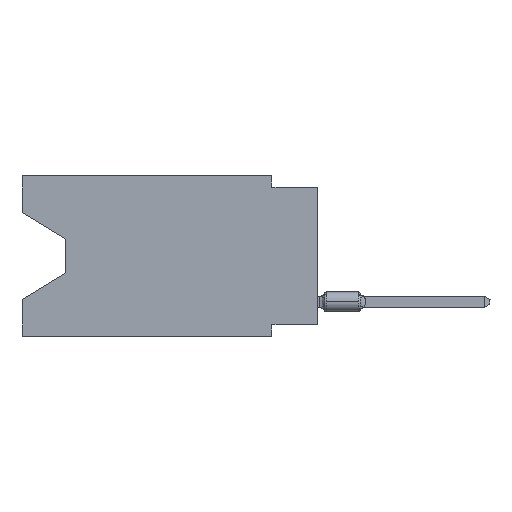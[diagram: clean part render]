
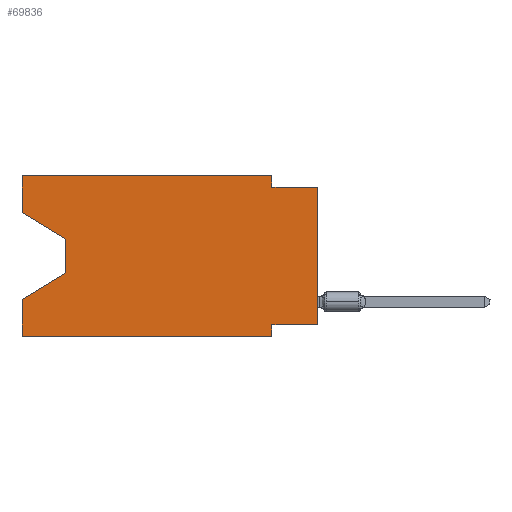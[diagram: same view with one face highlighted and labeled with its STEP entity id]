
A CAD part, left-side view. The second image highlights one B-rep face of the part: STEP entity #69836.
In plain terms, the highlighted planar face has unit normal (-1, 0, 0).
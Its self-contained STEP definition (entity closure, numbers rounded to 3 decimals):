
#1638 = CARTESIAN_POINT ( 'NONE',  ( 0., 13.97, -5.385 ) ) ;
#1983 = EDGE_CURVE ( 'NONE', #55844, #49080, #40251, .T. ) ;
#2470 = VERTEX_POINT ( 'NONE', #75733 ) ;
#3152 = VECTOR ( 'NONE', #27946, 1000. ) ;
#5003 = FACE_OUTER_BOUND ( 'NONE', #27251, .T. ) ;
#5547 = CARTESIAN_POINT ( 'NONE',  ( 0., 16.383, 0. ) ) ;
#6518 = CARTESIAN_POINT ( 'NONE',  ( 0., 2.54, -0.635 ) ) ;
#8444 = CARTESIAN_POINT ( 'NONE',  ( 0., 0., 0. ) ) ;
#10060 = DIRECTION ( 'NONE',  ( 0., 0., 1. ) ) ;
#11583 = VERTEX_POINT ( 'NONE', #1638 ) ;
#13618 = ORIENTED_EDGE ( 'NONE', *, *, #90701, .T. ) ;
#14977 = VECTOR ( 'NONE', #93194, 1000. ) ;
#16035 = DIRECTION ( 'NONE',  ( 0., 0.855, -0.519 ) ) ;
#16359 = LINE ( 'NONE', #57044, #100465 ) ;
#16659 = CARTESIAN_POINT ( 'NONE',  ( 0., 16.383, 0. ) ) ;
#18614 = DIRECTION ( 'NONE',  ( 0., 0., -1. ) ) ;
#20762 = ORIENTED_EDGE ( 'NONE', *, *, #57375, .F. ) ;
#21082 = ORIENTED_EDGE ( 'NONE', *, *, #100007, .T. ) ;
#21471 = VERTEX_POINT ( 'NONE', #67678 ) ;
#24738 = CARTESIAN_POINT ( 'NONE',  ( 0., 16.383, -6.852 ) ) ;
#27251 = EDGE_LOOP ( 'NONE', ( #30682, #13618, #50802, #34858, #59614, #75431, #28602, #21082, #20762, #68405, #90600, #79292 ) ) ;
#27256 = VECTOR ( 'NONE', #62671, 1000. ) ;
#27274 = VECTOR ( 'NONE', #16035, 1000. ) ;
#27509 = DIRECTION ( 'NONE',  ( 0., -1., 0. ) ) ;
#27946 = DIRECTION ( 'NONE',  ( 0., 0., -1. ) ) ;
#28602 = ORIENTED_EDGE ( 'NONE', *, *, #46644, .F. ) ;
#29047 = LINE ( 'NONE', #37188, #27256 ) ;
#29866 = VERTEX_POINT ( 'NONE', #24738 ) ;
#30682 = ORIENTED_EDGE ( 'NONE', *, *, #77262, .T. ) ;
#30712 = EDGE_CURVE ( 'NONE', #11583, #29866, #32278, .T. ) ;
#31211 = AXIS2_PLACEMENT_3D ( 'NONE', #5547, #45135, #95024 ) ;
#31554 = DIRECTION ( 'NONE',  ( 0., -0.855, -0.519 ) ) ;
#32278 = LINE ( 'NONE', #71374, #27274 ) ;
#34543 = VECTOR ( 'NONE', #27509, 1000. ) ;
#34858 = ORIENTED_EDGE ( 'NONE', *, *, #101920, .F. ) ;
#35839 = CARTESIAN_POINT ( 'NONE',  ( 0., 16.383, 0. ) ) ;
#35952 = LINE ( 'NONE', #75556, #74401 ) ;
#37188 = CARTESIAN_POINT ( 'NONE',  ( 0., 0., -8.255 ) ) ;
#37203 = VERTEX_POINT ( 'NONE', #104603 ) ;
#37918 = EDGE_CURVE ( 'NONE', #37203, #92675, #44740, .T. ) ;
#40251 = LINE ( 'NONE', #82004, #14977 ) ;
#42474 = VECTOR ( 'NONE', #84125, 1000. ) ;
#42862 = CARTESIAN_POINT ( 'NONE',  ( 0., 13.97, -3.505 ) ) ;
#43142 = LINE ( 'NONE', #59421, #3152 ) ;
#43852 = VERTEX_POINT ( 'NONE', #97502 ) ;
#44740 = LINE ( 'NONE', #84344, #86410 ) ;
#45135 = DIRECTION ( 'NONE',  ( 1., 0., 0. ) ) ;
#46117 = EDGE_CURVE ( 'NONE', #92675, #43852, #71079, .T. ) ;
#46644 = EDGE_CURVE ( 'NONE', #90921, #55844, #29047, .T. ) ;
#48182 = DIRECTION ( 'NONE',  ( 0., 0., 1. ) ) ;
#49080 = VERTEX_POINT ( 'NONE', #61221 ) ;
#50802 = ORIENTED_EDGE ( 'NONE', *, *, #30712, .T. ) ;
#51045 = CARTESIAN_POINT ( 'NONE',  ( 0., 0., -0.635 ) ) ;
#54368 = CARTESIAN_POINT ( 'NONE',  ( 0., 2.54, -8.255 ) ) ;
#55844 = VERTEX_POINT ( 'NONE', #54368 ) ;
#57044 = CARTESIAN_POINT ( 'NONE',  ( 0., 16.383, -2.038 ) ) ;
#57375 = EDGE_CURVE ( 'NONE', #92942, #21471, #84660, .T. ) ;
#59421 = CARTESIAN_POINT ( 'NONE',  ( 0., 13.97, -3.505 ) ) ;
#59614 = ORIENTED_EDGE ( 'NONE', *, *, #69388, .T. ) ;
#61221 = CARTESIAN_POINT ( 'NONE',  ( 0., 2.54, -8.89 ) ) ;
#62671 = DIRECTION ( 'NONE',  ( 0., 1., 0. ) ) ;
#65808 = VECTOR ( 'NONE', #48182, 1000. ) ;
#67678 = CARTESIAN_POINT ( 'NONE',  ( 0., 0., -0.635 ) ) ;
#68405 = ORIENTED_EDGE ( 'NONE', *, *, #76945, .F. ) ;
#69388 = EDGE_CURVE ( 'NONE', #2470, #49080, #70869, .T. ) ;
#69836 = ADVANCED_FACE ( 'NONE', ( #5003 ), #103671, .F. ) ;
#70869 = LINE ( 'NONE', #79549, #34543 ) ;
#71079 = LINE ( 'NONE', #16659, #101485 ) ;
#71374 = CARTESIAN_POINT ( 'NONE',  ( 0., 13.97, -5.385 ) ) ;
#71890 = VERTEX_POINT ( 'NONE', #42862 ) ;
#74401 = VECTOR ( 'NONE', #18614, 1000. ) ;
#74601 = DIRECTION ( 'NONE',  ( 0., 0., 1. ) ) ;
#75431 = ORIENTED_EDGE ( 'NONE', *, *, #1983, .F. ) ;
#75556 = CARTESIAN_POINT ( 'NONE',  ( 0., 2.54, 0. ) ) ;
#75733 = CARTESIAN_POINT ( 'NONE',  ( 0., 16.383, -8.89 ) ) ;
#76945 = EDGE_CURVE ( 'NONE', #43852, #92942, #35952, .T. ) ;
#77262 = EDGE_CURVE ( 'NONE', #37203, #71890, #16359, .T. ) ;
#79292 = ORIENTED_EDGE ( 'NONE', *, *, #37918, .F. ) ;
#79549 = CARTESIAN_POINT ( 'NONE',  ( 0., 16.383, -8.89 ) ) ;
#82004 = CARTESIAN_POINT ( 'NONE',  ( 0., 2.54, -8.89 ) ) ;
#82646 = CARTESIAN_POINT ( 'NONE',  ( 0., 0., -8.255 ) ) ;
#84125 = DIRECTION ( 'NONE',  ( 0., -1., 0. ) ) ;
#84344 = CARTESIAN_POINT ( 'NONE',  ( 0., 16.383, 0. ) ) ;
#84660 = LINE ( 'NONE', #51045, #42474 ) ;
#86410 = VECTOR ( 'NONE', #10060, 1000. ) ;
#90600 = ORIENTED_EDGE ( 'NONE', *, *, #46117, .F. ) ;
#90701 = EDGE_CURVE ( 'NONE', #71890, #11583, #43142, .T. ) ;
#90921 = VERTEX_POINT ( 'NONE', #82646 ) ;
#92675 = VERTEX_POINT ( 'NONE', #35839 ) ;
#92942 = VERTEX_POINT ( 'NONE', #6518 ) ;
#93194 = DIRECTION ( 'NONE',  ( 0., 0., -1. ) ) ;
#95024 = DIRECTION ( 'NONE',  ( 0., 0., -1. ) ) ;
#97502 = CARTESIAN_POINT ( 'NONE',  ( 0., 2.54, 0. ) ) ;
#99607 = DIRECTION ( 'NONE',  ( 0., -1., 0. ) ) ;
#100007 = EDGE_CURVE ( 'NONE', #90921, #21471, #107133, .T. ) ;
#100088 = VECTOR ( 'NONE', #74601, 1000. ) ;
#100465 = VECTOR ( 'NONE', #31554, 1000. ) ;
#101485 = VECTOR ( 'NONE', #99607, 1000. ) ;
#101920 = EDGE_CURVE ( 'NONE', #2470, #29866, #106728, .T. ) ;
#103671 = PLANE ( 'NONE',  #31211 ) ;
#104603 = CARTESIAN_POINT ( 'NONE',  ( 0., 16.383, -2.038 ) ) ;
#105123 = CARTESIAN_POINT ( 'NONE',  ( 0., 16.383, 0. ) ) ;
#106728 = LINE ( 'NONE', #105123, #65808 ) ;
#107133 = LINE ( 'NONE', #8444, #100088 ) ;
